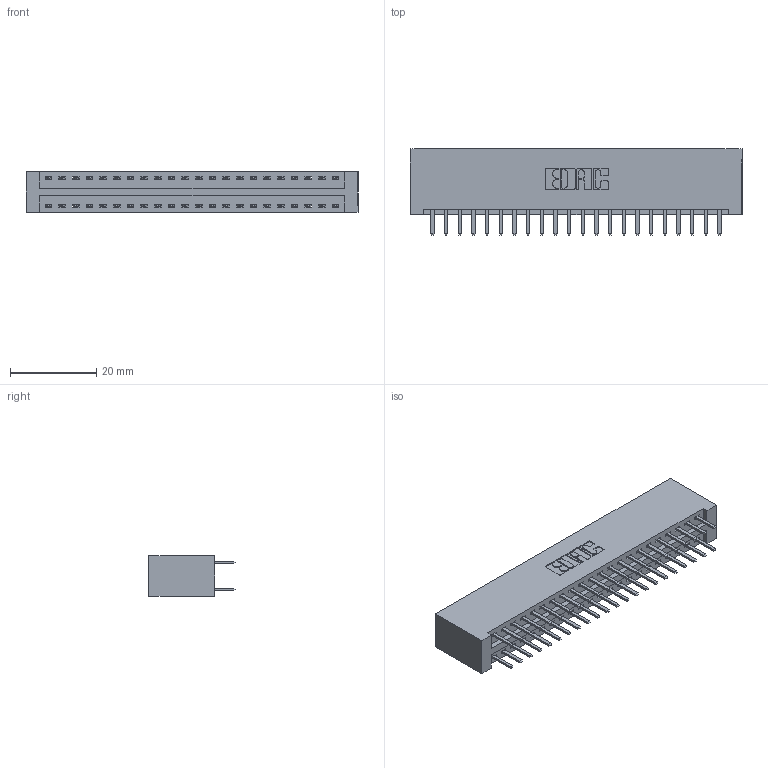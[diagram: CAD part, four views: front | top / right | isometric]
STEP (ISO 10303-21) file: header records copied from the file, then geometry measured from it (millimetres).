
FILE_DESCRIPTION (( 'STEP AP203' ), '1' );
FILE_NAME ('396-044-520-201.STEP', '2019-10-30T11:15:51', ( '' ), ( '' ), 'SwSTEP 2.0', 'SolidWorks 2016', '' );
FILE_SCHEMA (( 'CONFIG_CONTROL_DESIGN' ));
Length unit declared in the file: inch
Products named in the file (3): 396-044-520-201; 345-292-001_345-293-120; 346 Part_No Mounting Lugs
Assembly tree (45 placements, depth 2):
  396-044-520-201
    346 Part_No Mounting Lugs
    345-292-001_345-293-120  x44
Bounding box: 77.09 x 20.02 x 9.4 mm (x, y, z)
Volume: 7915.7 mm3; surface area: 10684.2 mm2
Topology: 45 solids, 45 shells, 2578 faces, 7477 edges, 4866 vertices
Faces by surface type: plane 1700, cylinder 878
Entity records: 16887 total; most frequent: CARTESIAN_POINT 2820, ORIENTED_EDGE 2742, DIRECTION 2519, EDGE_CURVE 1371, LINE 1155, VECTOR 1155, VERTEX_POINT 910, AXIS2_PLACEMENT_3D 682
